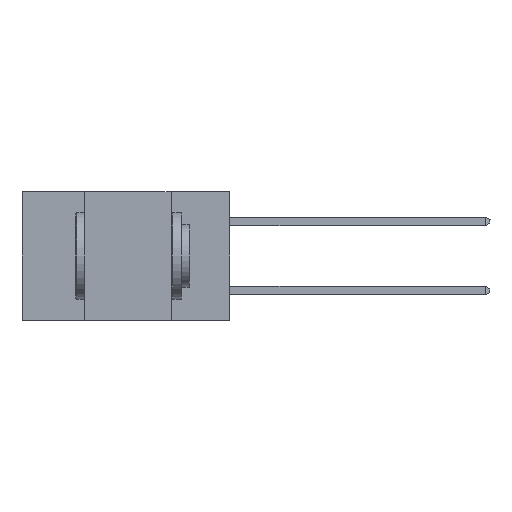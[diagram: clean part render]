
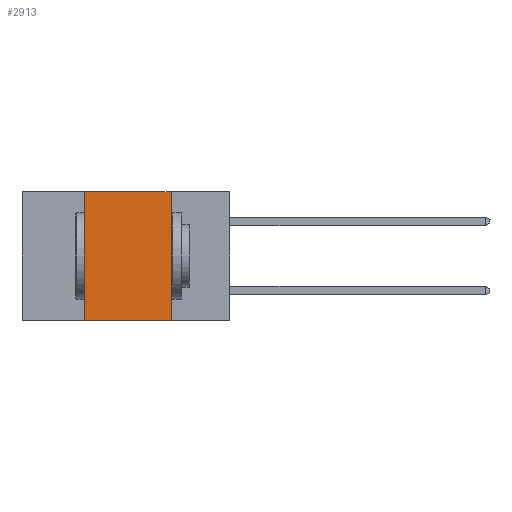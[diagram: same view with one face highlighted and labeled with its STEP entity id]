
A CAD part, left-side view. The second image highlights one B-rep face of the part: STEP entity #2913.
In plain terms, the highlighted planar face has unit normal (-1, 0, 0).
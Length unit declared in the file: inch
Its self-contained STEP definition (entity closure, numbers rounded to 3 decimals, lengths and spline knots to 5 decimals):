
#494 = EDGE_CURVE ( 'NONE', #9973, #5705, #10663, .T. ) ;
#824 = VERTEX_POINT ( 'NONE', #7906 ) ;
#1767 = PLANE ( 'NONE',  #2511 ) ;
#1920 = DIRECTION ( 'NONE',  ( 0., -1., 0. ) ) ;
#2511 = AXIS2_PLACEMENT_3D ( 'NONE', #4781, #11233, #3718 ) ;
#2633 = EDGE_LOOP ( 'NONE', ( #5228, #5950, #4593, #11426 ) ) ;
#2913 = ADVANCED_FACE ( 'NONE', ( #4369 ), #1767, .F. ) ;
#3011 = LINE ( 'NONE', #10821, #5323 ) ;
#3718 = DIRECTION ( 'NONE',  ( 0., 0., -1. ) ) ;
#4024 = CARTESIAN_POINT ( 'NONE',  ( 0., 0.42, -0.37 ) ) ;
#4369 = FACE_OUTER_BOUND ( 'NONE', #2633, .T. ) ;
#4593 = ORIENTED_EDGE ( 'NONE', *, *, #494, .F. ) ;
#4755 = LINE ( 'NONE', #10391, #11004 ) ;
#4781 = CARTESIAN_POINT ( 'NONE',  ( 0., 0.6, 0. ) ) ;
#4860 = VECTOR ( 'NONE', #6968, 39.37008 ) ;
#5006 = EDGE_CURVE ( 'NONE', #9973, #824, #4755, .T. ) ;
#5228 = ORIENTED_EDGE ( 'NONE', *, *, #6029, .F. ) ;
#5323 = VECTOR ( 'NONE', #10571, 39.37008 ) ;
#5705 = VERTEX_POINT ( 'NONE', #6285 ) ;
#5950 = ORIENTED_EDGE ( 'NONE', *, *, #6556, .F. ) ;
#6029 = EDGE_CURVE ( 'NONE', #10569, #824, #8898, .T. ) ;
#6285 = CARTESIAN_POINT ( 'NONE',  ( 0., 0.42, 0. ) ) ;
#6547 = CARTESIAN_POINT ( 'NONE',  ( 0., 0.42, -0.37 ) ) ;
#6556 = EDGE_CURVE ( 'NONE', #5705, #10569, #3011, .T. ) ;
#6968 = DIRECTION ( 'NONE',  ( 0., 0., 1. ) ) ;
#7815 = CARTESIAN_POINT ( 'NONE',  ( 0., 0.17, -0.37 ) ) ;
#7906 = CARTESIAN_POINT ( 'NONE',  ( 0., 0.17, -0.37 ) ) ;
#8002 = DIRECTION ( 'NONE',  ( 0., 0., -1. ) ) ;
#8898 = LINE ( 'NONE', #7815, #11638 ) ;
#9080 = CARTESIAN_POINT ( 'NONE',  ( 0., 0.17, 0. ) ) ;
#9973 = VERTEX_POINT ( 'NONE', #6547 ) ;
#10391 = CARTESIAN_POINT ( 'NONE',  ( 0., 0.6, -0.37 ) ) ;
#10569 = VERTEX_POINT ( 'NONE', #9080 ) ;
#10571 = DIRECTION ( 'NONE',  ( 0., -1., 0. ) ) ;
#10663 = LINE ( 'NONE', #4024, #4860 ) ;
#10821 = CARTESIAN_POINT ( 'NONE',  ( 0., 0.6, 0. ) ) ;
#11004 = VECTOR ( 'NONE', #1920, 39.37008 ) ;
#11233 = DIRECTION ( 'NONE',  ( 1., 0., 0. ) ) ;
#11426 = ORIENTED_EDGE ( 'NONE', *, *, #5006, .T. ) ;
#11638 = VECTOR ( 'NONE', #8002, 39.37008 ) ;
